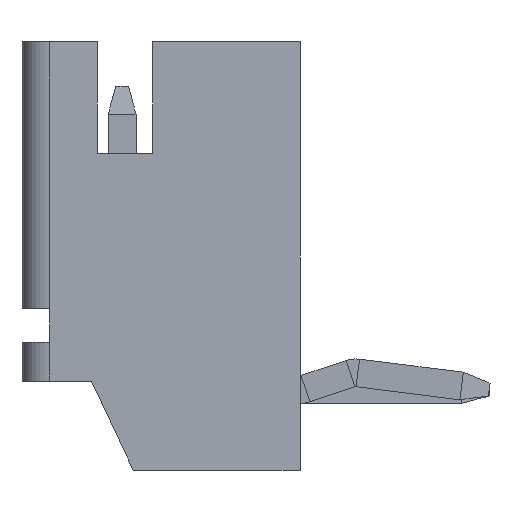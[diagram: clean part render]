
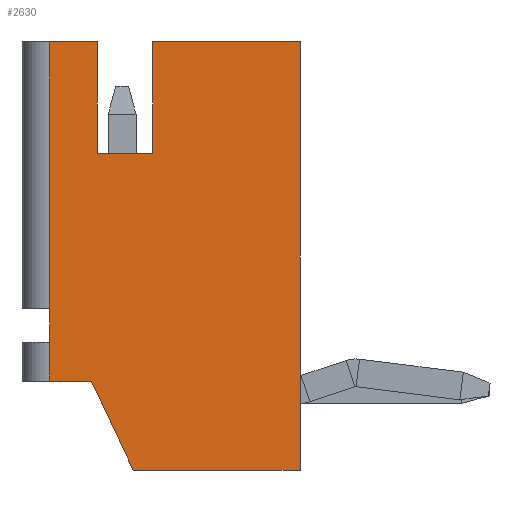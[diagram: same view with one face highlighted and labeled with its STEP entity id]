
A CAD part, left-side view. The second image highlights one B-rep face of the part: STEP entity #2630.
In plain terms, the highlighted planar face has unit normal (-1, 0, 0).
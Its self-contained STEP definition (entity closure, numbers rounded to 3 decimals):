
#17 = VERTEX_POINT ( 'NONE', #3777 ) ;
#20 = EDGE_CURVE ( 'NONE', #17, #952, #2664, .T. ) ;
#72 = LINE ( 'NONE', #532, #1570 ) ;
#126 = ORIENTED_EDGE ( 'NONE', *, *, #3569, .T. ) ;
#277 = DIRECTION ( 'NONE',  ( 0., 1., 0. ) ) ;
#372 = VERTEX_POINT ( 'NONE', #3907 ) ;
#436 = LINE ( 'NONE', #2633, #3507 ) ;
#532 = CARTESIAN_POINT ( 'NONE',  ( -2., -3.2, -1.6 ) ) ;
#563 = CARTESIAN_POINT ( 'NONE',  ( -2., -3.2, -1.6 ) ) ;
#568 = LINE ( 'NONE', #886, #1463 ) ;
#589 = DIRECTION ( 'NONE',  ( 0., 0., -1. ) ) ;
#611 = VECTOR ( 'NONE', #1217, 1000. ) ;
#664 = ORIENTED_EDGE ( 'NONE', *, *, #2669, .T. ) ;
#705 = CARTESIAN_POINT ( 'NONE',  ( -2., -0.55, 6.1 ) ) ;
#744 = LINE ( 'NONE', #1409, #2997 ) ;
#753 = LINE ( 'NONE', #1519, #2583 ) ;
#792 = CARTESIAN_POINT ( 'NONE',  ( -2., -0.2, -1.6 ) ) ;
#798 = EDGE_CURVE ( 'NONE', #3774, #954, #72, .T. ) ;
#803 = DIRECTION ( 'NONE',  ( 0., 0., -1. ) ) ;
#856 = DIRECTION ( 'NONE',  ( 0., -0.424, -0.905 ) ) ;
#870 = ORIENTED_EDGE ( 'NONE', *, *, #20, .T. ) ;
#886 = CARTESIAN_POINT ( 'NONE',  ( -2., -3.2, 6.1 ) ) ;
#909 = EDGE_CURVE ( 'NONE', #372, #4540, #2982, .T. ) ;
#923 = DIRECTION ( 'NONE',  ( 0., -1., 0. ) ) ;
#952 = VERTEX_POINT ( 'NONE', #3586 ) ;
#954 = VERTEX_POINT ( 'NONE', #563 ) ;
#1100 = EDGE_LOOP ( 'NONE', ( #1363, #2860, #2345, #4218, #1971, #4105, #664, #3082, #3726, #4195, #126, #870 ) ) ;
#1217 = DIRECTION ( 'NONE',  ( 0., -1., 0. ) ) ;
#1319 = LINE ( 'NONE', #2789, #611 ) ;
#1363 = ORIENTED_EDGE ( 'NONE', *, *, #2231, .T. ) ;
#1409 = CARTESIAN_POINT ( 'NONE',  ( -2., -0.55, 6.1 ) ) ;
#1422 = PLANE ( 'NONE',  #3246 ) ;
#1444 = VERTEX_POINT ( 'NONE', #2247 ) ;
#1463 = VECTOR ( 'NONE', #2417, 1000. ) ;
#1519 = CARTESIAN_POINT ( 'NONE',  ( -2., 0.45, 4.1 ) ) ;
#1536 = VERTEX_POINT ( 'NONE', #1901 ) ;
#1570 = VECTOR ( 'NONE', #923, 1000. ) ;
#1653 = LINE ( 'NONE', #792, #3239 ) ;
#1722 = DIRECTION ( 'NONE',  ( 0., -1., 0. ) ) ;
#1744 = VECTOR ( 'NONE', #1838, 1000. ) ;
#1824 = CARTESIAN_POINT ( 'NONE',  ( -2., -0.55, 6.1 ) ) ;
#1838 = DIRECTION ( 'NONE',  ( 0., 0., -1. ) ) ;
#1881 = EDGE_CURVE ( 'NONE', #2452, #3397, #753, .T. ) ;
#1901 = CARTESIAN_POINT ( 'NONE',  ( -2., -3.2, 6.1 ) ) ;
#1971 = ORIENTED_EDGE ( 'NONE', *, *, #798, .T. ) ;
#2231 = EDGE_CURVE ( 'NONE', #952, #372, #4736, .T. ) ;
#2247 = CARTESIAN_POINT ( 'NONE',  ( -2., 0.55, 0. ) ) ;
#2311 = EDGE_CURVE ( 'NONE', #954, #1536, #568, .T. ) ;
#2345 = ORIENTED_EDGE ( 'NONE', *, *, #3456, .T. ) ;
#2367 = DIRECTION ( 'NONE',  ( 0., 0., -1. ) ) ;
#2417 = DIRECTION ( 'NONE',  ( 0., 0., 1. ) ) ;
#2452 = VERTEX_POINT ( 'NONE', #4820 ) ;
#2580 = CARTESIAN_POINT ( 'NONE',  ( -2., 0.45, 6.1 ) ) ;
#2583 = VECTOR ( 'NONE', #3027, 1000. ) ;
#2630 = ADVANCED_FACE ( 'NONE', ( #4438 ), #1422, .T. ) ;
#2633 = CARTESIAN_POINT ( 'NONE',  ( -2., 0.45, 6.1 ) ) ;
#2664 = LINE ( 'NONE', #4472, #3016 ) ;
#2669 = EDGE_CURVE ( 'NONE', #1536, #4530, #744, .T. ) ;
#2782 = CARTESIAN_POINT ( 'NONE',  ( -2., 1.3, 1.3 ) ) ;
#2789 = CARTESIAN_POINT ( 'NONE',  ( -2., 1.8, 0. ) ) ;
#2859 = CARTESIAN_POINT ( 'NONE',  ( -2., 1.3, 0. ) ) ;
#2860 = ORIENTED_EDGE ( 'NONE', *, *, #909, .T. ) ;
#2982 = LINE ( 'NONE', #2859, #4015 ) ;
#2997 = VECTOR ( 'NONE', #277, 1000. ) ;
#3016 = VECTOR ( 'NONE', #803, 1000. ) ;
#3027 = DIRECTION ( 'NONE',  ( 0., 1., 0. ) ) ;
#3033 = CARTESIAN_POINT ( 'NONE',  ( -2., 1.3, 0. ) ) ;
#3063 = EDGE_CURVE ( 'NONE', #4530, #2452, #4788, .T. ) ;
#3082 = ORIENTED_EDGE ( 'NONE', *, *, #3063, .T. ) ;
#3110 = EDGE_CURVE ( 'NONE', #3397, #3146, #436, .T. ) ;
#3146 = VERTEX_POINT ( 'NONE', #2580 ) ;
#3226 = VECTOR ( 'NONE', #2367, 1000. ) ;
#3239 = VECTOR ( 'NONE', #856, 1000. ) ;
#3246 = AXIS2_PLACEMENT_3D ( 'NONE', #3673, #4004, #1722 ) ;
#3397 = VERTEX_POINT ( 'NONE', #3523 ) ;
#3456 = EDGE_CURVE ( 'NONE', #4540, #1444, #1319, .T. ) ;
#3507 = VECTOR ( 'NONE', #4827, 1000. ) ;
#3523 = CARTESIAN_POINT ( 'NONE',  ( -2., 0.45, 4.1 ) ) ;
#3569 = EDGE_CURVE ( 'NONE', #3146, #17, #4199, .T. ) ;
#3582 = DIRECTION ( 'NONE',  ( 0., 1., 0. ) ) ;
#3586 = CARTESIAN_POINT ( 'NONE',  ( -2., 1.3, 1.3 ) ) ;
#3673 = CARTESIAN_POINT ( 'NONE',  ( -2., 0., 0. ) ) ;
#3726 = ORIENTED_EDGE ( 'NONE', *, *, #1881, .T. ) ;
#3774 = VERTEX_POINT ( 'NONE', #4724 ) ;
#3777 = CARTESIAN_POINT ( 'NONE',  ( -2., 1.3, 6.1 ) ) ;
#3907 = CARTESIAN_POINT ( 'NONE',  ( -2., 1.3, 0.7 ) ) ;
#3940 = CARTESIAN_POINT ( 'NONE',  ( -2., 1.8, 6.1 ) ) ;
#4004 = DIRECTION ( 'NONE',  ( -1., 0., 0. ) ) ;
#4015 = VECTOR ( 'NONE', #589, 1000. ) ;
#4105 = ORIENTED_EDGE ( 'NONE', *, *, #2311, .T. ) ;
#4195 = ORIENTED_EDGE ( 'NONE', *, *, #3110, .T. ) ;
#4199 = LINE ( 'NONE', #3940, #4484 ) ;
#4218 = ORIENTED_EDGE ( 'NONE', *, *, #4834, .T. ) ;
#4438 = FACE_OUTER_BOUND ( 'NONE', #1100, .T. ) ;
#4472 = CARTESIAN_POINT ( 'NONE',  ( -2., 1.3, 0. ) ) ;
#4484 = VECTOR ( 'NONE', #3582, 1000. ) ;
#4530 = VERTEX_POINT ( 'NONE', #705 ) ;
#4540 = VERTEX_POINT ( 'NONE', #3033 ) ;
#4724 = CARTESIAN_POINT ( 'NONE',  ( -2., -0.2, -1.6 ) ) ;
#4736 = LINE ( 'NONE', #2782, #3226 ) ;
#4788 = LINE ( 'NONE', #1824, #1744 ) ;
#4820 = CARTESIAN_POINT ( 'NONE',  ( -2., -0.55, 4.1 ) ) ;
#4827 = DIRECTION ( 'NONE',  ( 0., 0., 1. ) ) ;
#4834 = EDGE_CURVE ( 'NONE', #1444, #3774, #1653, .T. ) ;
